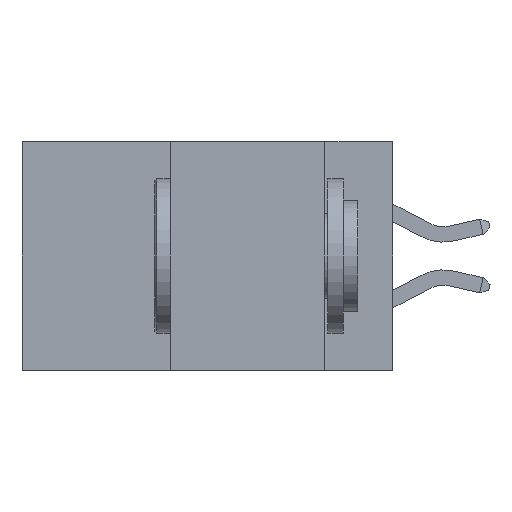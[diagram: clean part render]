
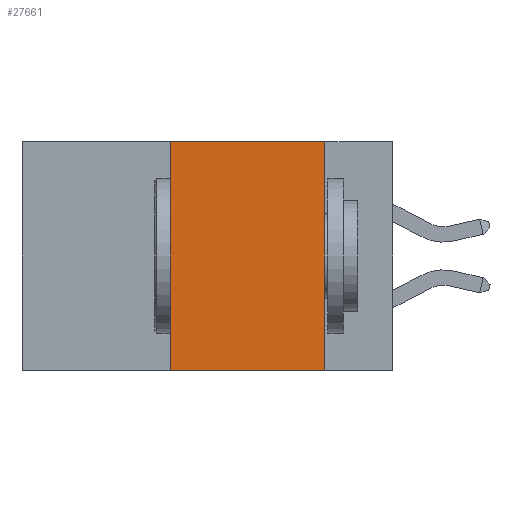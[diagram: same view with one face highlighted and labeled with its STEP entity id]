
A CAD part, left-side view. The second image highlights one B-rep face of the part: STEP entity #27661.
In plain terms, the highlighted planar face has unit normal (-1, 0, 0).
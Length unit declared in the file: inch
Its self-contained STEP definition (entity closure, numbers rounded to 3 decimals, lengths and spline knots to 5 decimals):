
#352 = DIRECTION ( 'NONE',  ( 0., -1., 0. ) ) ;
#786 = CARTESIAN_POINT ( 'NONE',  ( 0., 0.6, 0. ) ) ;
#1019 = DIRECTION ( 'NONE',  ( 0., 0., -1. ) ) ;
#2517 = VERTEX_POINT ( 'NONE', #6255 ) ;
#4566 = EDGE_CURVE ( 'NONE', #7099, #9025, #8701, .T. ) ;
#5046 = CARTESIAN_POINT ( 'NONE',  ( 0., 0.6, 0. ) ) ;
#6255 = CARTESIAN_POINT ( 'NONE',  ( 0., 0.36, 0. ) ) ;
#6287 = ORIENTED_EDGE ( 'NONE', *, *, #4566, .F. ) ;
#6339 = CARTESIAN_POINT ( 'NONE',  ( 0., 0.6, -0.37 ) ) ;
#7099 = VERTEX_POINT ( 'NONE', #20152 ) ;
#7224 = CARTESIAN_POINT ( 'NONE',  ( 0., 0.36, -0.37 ) ) ;
#8461 = CARTESIAN_POINT ( 'NONE',  ( 0., 0.36, 0. ) ) ;
#8701 = LINE ( 'NONE', #27025, #21606 ) ;
#8979 = LINE ( 'NONE', #8461, #22248 ) ;
#9025 = VERTEX_POINT ( 'NONE', #26952 ) ;
#9671 = DIRECTION ( 'NONE',  ( 0., 0., -1. ) ) ;
#11489 = ORIENTED_EDGE ( 'NONE', *, *, #16395, .F. ) ;
#12139 = AXIS2_PLACEMENT_3D ( 'NONE', #786, #18369, #9671 ) ;
#13445 = VECTOR ( 'NONE', #17910, 39.37008 ) ;
#14822 = ORIENTED_EDGE ( 'NONE', *, *, #19411, .T. ) ;
#16395 = EDGE_CURVE ( 'NONE', #2517, #7099, #27377, .T. ) ;
#16889 = ORIENTED_EDGE ( 'NONE', *, *, #26096, .F. ) ;
#17179 = DIRECTION ( 'NONE',  ( 0., 0., 1. ) ) ;
#17267 = EDGE_LOOP ( 'NONE', ( #6287, #11489, #16889, #14822 ) ) ;
#17910 = DIRECTION ( 'NONE',  ( 0., -1., 0. ) ) ;
#18369 = DIRECTION ( 'NONE',  ( 1., 0., 0. ) ) ;
#18703 = VERTEX_POINT ( 'NONE', #7224 ) ;
#19411 = EDGE_CURVE ( 'NONE', #18703, #9025, #24533, .T. ) ;
#20152 = CARTESIAN_POINT ( 'NONE',  ( 0., 0.11, 0. ) ) ;
#21606 = VECTOR ( 'NONE', #1019, 39.37008 ) ;
#22248 = VECTOR ( 'NONE', #17179, 39.37008 ) ;
#24206 = VECTOR ( 'NONE', #352, 39.37008 ) ;
#24533 = LINE ( 'NONE', #6339, #24206 ) ;
#24999 = PLANE ( 'NONE',  #12139 ) ;
#25173 = FACE_OUTER_BOUND ( 'NONE', #17267, .T. ) ;
#26096 = EDGE_CURVE ( 'NONE', #18703, #2517, #8979, .T. ) ;
#26952 = CARTESIAN_POINT ( 'NONE',  ( 0., 0.11, -0.37 ) ) ;
#27025 = CARTESIAN_POINT ( 'NONE',  ( 0., 0.11, 0. ) ) ;
#27377 = LINE ( 'NONE', #5046, #13445 ) ;
#27661 = ADVANCED_FACE ( 'NONE', ( #25173 ), #24999, .F. ) ;
